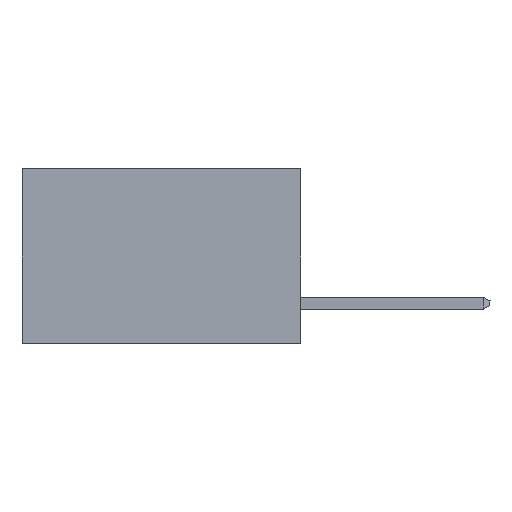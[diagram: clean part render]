
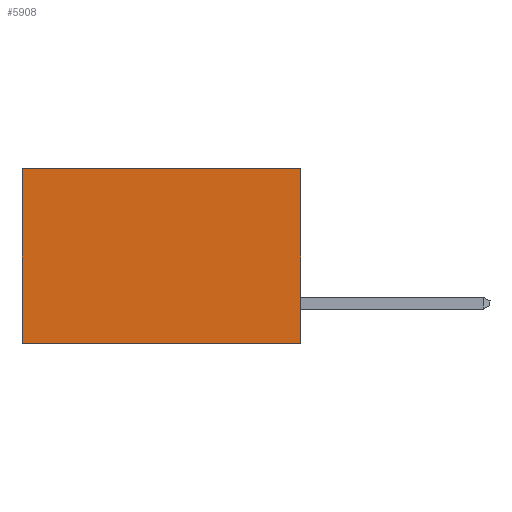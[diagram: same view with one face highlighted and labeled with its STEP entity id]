
A CAD part, left-side view. The second image highlights one B-rep face of the part: STEP entity #5908.
In plain terms, the highlighted planar face has unit normal (-1, 0, 0).
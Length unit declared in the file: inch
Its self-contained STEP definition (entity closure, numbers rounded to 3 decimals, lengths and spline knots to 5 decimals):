
#54 = DIRECTION ( 'NONE',  ( 0., 0., -1. ) ) ;
#146 = DIRECTION ( 'NONE',  ( 0., 1., 0. ) ) ;
#151 = LINE ( 'NONE', #9713, #6480 ) ;
#167 = DIRECTION ( 'NONE',  ( 0., 0., -1. ) ) ;
#989 = EDGE_CURVE ( 'NONE', #4152, #3768, #7243, .T. ) ;
#1768 = CARTESIAN_POINT ( 'NONE',  ( 0.277, 0., -0.37 ) ) ;
#2141 = EDGE_CURVE ( 'NONE', #2304, #9390, #9329, .T. ) ;
#2304 = VERTEX_POINT ( 'NONE', #4880 ) ;
#2436 = CARTESIAN_POINT ( 'NONE',  ( 0.277, 0.59, -0.37 ) ) ;
#2688 = CARTESIAN_POINT ( 'NONE',  ( 0.277, 0.59, 0. ) ) ;
#2698 = DIRECTION ( 'NONE',  ( 0., 1., 0. ) ) ;
#2986 = DIRECTION ( 'NONE',  ( 0., 0., -1. ) ) ;
#3768 = VERTEX_POINT ( 'NONE', #2436 ) ;
#4027 = EDGE_LOOP ( 'NONE', ( #5994, #5198, #6466, #6727 ) ) ;
#4076 = LINE ( 'NONE', #1768, #7844 ) ;
#4152 = VERTEX_POINT ( 'NONE', #2688 ) ;
#4183 = EDGE_CURVE ( 'NONE', #2304, #4152, #151, .T. ) ;
#4587 = DIRECTION ( 'NONE',  ( 1., 0., 0. ) ) ;
#4823 = EDGE_CURVE ( 'NONE', #9390, #3768, #4076, .T. ) ;
#4880 = CARTESIAN_POINT ( 'NONE',  ( 0.277, 0., 0. ) ) ;
#5190 = CARTESIAN_POINT ( 'NONE',  ( 0.277, 0., -0.37 ) ) ;
#5198 = ORIENTED_EDGE ( 'NONE', *, *, #4823, .F. ) ;
#5272 = VECTOR ( 'NONE', #54, 39.37008 ) ;
#5348 = PLANE ( 'NONE',  #6558 ) ;
#5624 = CARTESIAN_POINT ( 'NONE',  ( 0.277, 0., -0.37 ) ) ;
#5908 = ADVANCED_FACE ( 'NONE', ( #6787 ), #5348, .F. ) ;
#5994 = ORIENTED_EDGE ( 'NONE', *, *, #989, .T. ) ;
#6466 = ORIENTED_EDGE ( 'NONE', *, *, #2141, .F. ) ;
#6480 = VECTOR ( 'NONE', #146, 39.37008 ) ;
#6558 = AXIS2_PLACEMENT_3D ( 'NONE', #6911, #4587, #167 ) ;
#6727 = ORIENTED_EDGE ( 'NONE', *, *, #4183, .T. ) ;
#6787 = FACE_OUTER_BOUND ( 'NONE', #4027, .T. ) ;
#6911 = CARTESIAN_POINT ( 'NONE',  ( 0.277, 0., -0.37 ) ) ;
#7243 = LINE ( 'NONE', #9296, #5272 ) ;
#7810 = VECTOR ( 'NONE', #2986, 39.37008 ) ;
#7844 = VECTOR ( 'NONE', #2698, 39.37008 ) ;
#9296 = CARTESIAN_POINT ( 'NONE',  ( 0.277, 0.59, -0.37 ) ) ;
#9329 = LINE ( 'NONE', #5624, #7810 ) ;
#9390 = VERTEX_POINT ( 'NONE', #5190 ) ;
#9713 = CARTESIAN_POINT ( 'NONE',  ( 0.277, 0., 0. ) ) ;
